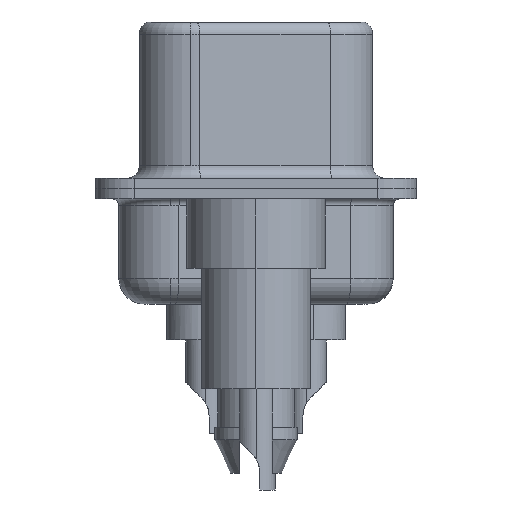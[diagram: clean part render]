
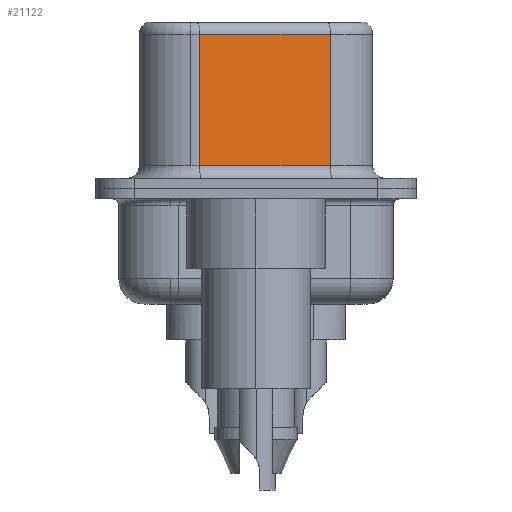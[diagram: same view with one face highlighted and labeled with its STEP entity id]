
A CAD part, left-side view. The second image highlights one B-rep face of the part: STEP entity #21122.
In plain terms, the highlighted planar face has unit normal (-0.985, -0.174, 0).
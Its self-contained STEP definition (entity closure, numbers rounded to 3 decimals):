
#1341 = DIRECTION ( 'NONE',  ( -0.174, 0.985, 0. ) ) ;
#3271 = ORIENTED_EDGE ( 'NONE', *, *, #23061, .T. ) ;
#3361 = VECTOR ( 'NONE', #3823, 1000. ) ;
#3823 = DIRECTION ( 'NONE',  ( 0., 0., -1. ) ) ;
#4013 = CARTESIAN_POINT ( 'NONE',  ( 4.58, -2.897, 0.9 ) ) ;
#6457 = VERTEX_POINT ( 'NONE', #8008 ) ;
#8008 = CARTESIAN_POINT ( 'NONE',  ( 4.58, -2.897, 6.02 ) ) ;
#9105 = LINE ( 'NONE', #16756, #3361 ) ;
#9564 = CARTESIAN_POINT ( 'NONE',  ( 4.58, -2.897, 6.02 ) ) ;
#10150 = LINE ( 'NONE', #10715, #15192 ) ;
#10202 = FACE_OUTER_BOUND ( 'NONE', #14075, .T. ) ;
#10715 = CARTESIAN_POINT ( 'NONE',  ( 4.58, -2.897, 6.52 ) ) ;
#10802 = LINE ( 'NONE', #4013, #21505 ) ;
#11736 = DIRECTION ( 'NONE',  ( -0.174, 0.985, 0. ) ) ;
#12799 = VECTOR ( 'NONE', #11736, 1000. ) ;
#13451 = ORIENTED_EDGE ( 'NONE', *, *, #20384, .T. ) ;
#13452 = LINE ( 'NONE', #9564, #12799 ) ;
#13810 = VERTEX_POINT ( 'NONE', #23268 ) ;
#14075 = EDGE_LOOP ( 'NONE', ( #26980, #13451, #3271, #27328 ) ) ;
#14321 = DIRECTION ( 'NONE',  ( 0.985, 0.174, 0. ) ) ;
#15192 = VECTOR ( 'NONE', #23485, 1000. ) ;
#16756 = CARTESIAN_POINT ( 'NONE',  ( 3.68, 2.203, 6.52 ) ) ;
#16842 = DIRECTION ( 'NONE',  ( 0.174, -0.985, 0. ) ) ;
#17316 = CARTESIAN_POINT ( 'NONE',  ( 4.58, -2.897, 0.9 ) ) ;
#18450 = EDGE_CURVE ( 'NONE', #24307, #21402, #10802, .T. ) ;
#18551 = CARTESIAN_POINT ( 'NONE',  ( 4.58, -2.897, 6.52 ) ) ;
#20384 = EDGE_CURVE ( 'NONE', #6457, #13810, #13452, .T. ) ;
#20692 = PLANE ( 'NONE',  #27173 ) ;
#21122 = ADVANCED_FACE ( 'NONE', ( #10202 ), #20692, .F. ) ;
#21402 = VERTEX_POINT ( 'NONE', #17316 ) ;
#21505 = VECTOR ( 'NONE', #16842, 1000. ) ;
#21927 = EDGE_CURVE ( 'NONE', #6457, #21402, #10150, .T. ) ;
#23061 = EDGE_CURVE ( 'NONE', #13810, #24307, #9105, .T. ) ;
#23268 = CARTESIAN_POINT ( 'NONE',  ( 3.68, 2.203, 6.02 ) ) ;
#23485 = DIRECTION ( 'NONE',  ( 0., 0., -1. ) ) ;
#24307 = VERTEX_POINT ( 'NONE', #26418 ) ;
#26418 = CARTESIAN_POINT ( 'NONE',  ( 3.68, 2.203, 0.9 ) ) ;
#26980 = ORIENTED_EDGE ( 'NONE', *, *, #21927, .F. ) ;
#27173 = AXIS2_PLACEMENT_3D ( 'NONE', #18551, #14321, #1341 ) ;
#27328 = ORIENTED_EDGE ( 'NONE', *, *, #18450, .T. ) ;
